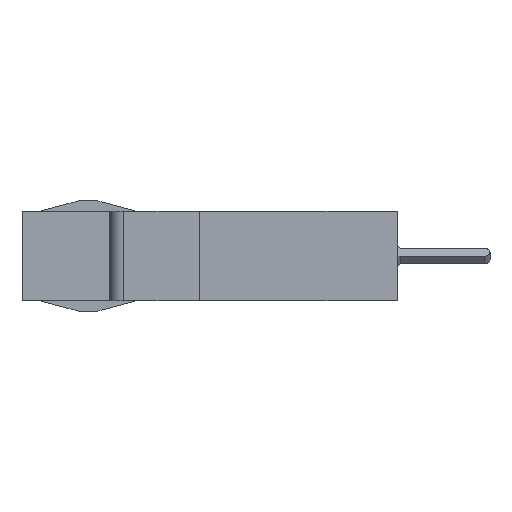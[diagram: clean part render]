
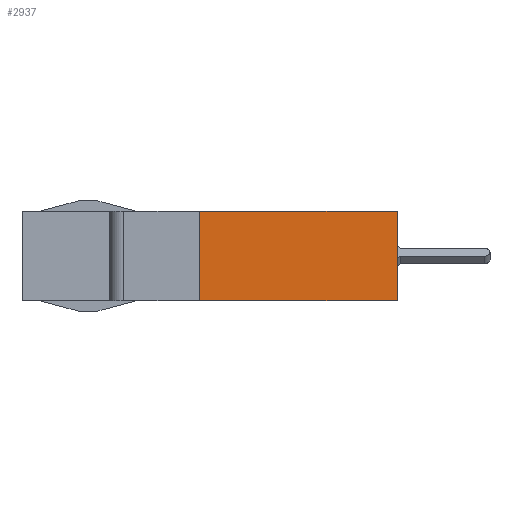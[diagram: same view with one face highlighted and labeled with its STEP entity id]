
A CAD part, left-side view. The second image highlights one B-rep face of the part: STEP entity #2937.
In plain terms, the highlighted planar face has unit normal (-1, 0, 0).
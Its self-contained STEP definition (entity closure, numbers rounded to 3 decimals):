
#182 = EDGE_CURVE ( 'NONE', #2905, #5426, #1135, .T. ) ;
#567 = DIRECTION ( 'NONE',  ( -1., 0., 0. ) ) ;
#622 = DIRECTION ( 'NONE',  ( 0., 0., 1. ) ) ;
#1115 = CARTESIAN_POINT ( 'NONE',  ( -2.235, 0., 2.54 ) ) ;
#1135 = LINE ( 'NONE', #4374, #2200 ) ;
#1329 = EDGE_CURVE ( 'NONE', #2905, #5324, #1978, .T. ) ;
#1419 = VECTOR ( 'NONE', #4460, 1000. ) ;
#1594 = DIRECTION ( 'NONE',  ( 0., 0., -1. ) ) ;
#1919 = CARTESIAN_POINT ( 'NONE',  ( -2.235, 0., -2.54 ) ) ;
#1951 = VERTEX_POINT ( 'NONE', #1115 ) ;
#1978 = LINE ( 'NONE', #3656, #1419 ) ;
#2200 = VECTOR ( 'NONE', #4913, 1000. ) ;
#2256 = EDGE_LOOP ( 'NONE', ( #5766, #2798, #2448, #4740 ) ) ;
#2448 = ORIENTED_EDGE ( 'NONE', *, *, #182, .F. ) ;
#2516 = EDGE_CURVE ( 'NONE', #5324, #1951, #4226, .T. ) ;
#2798 = ORIENTED_EDGE ( 'NONE', *, *, #5888, .T. ) ;
#2905 = VERTEX_POINT ( 'NONE', #5576 ) ;
#2937 = ADVANCED_FACE ( 'NONE', ( #6605 ), #5792, .T. ) ;
#3656 = CARTESIAN_POINT ( 'NONE',  ( -2.235, -11.176, -2.54 ) ) ;
#3705 = CARTESIAN_POINT ( 'NONE',  ( -2.235, -11.176, -2.54 ) ) ;
#4226 = LINE ( 'NONE', #4696, #4641 ) ;
#4374 = CARTESIAN_POINT ( 'NONE',  ( -2.235, -11.176, -2.54 ) ) ;
#4460 = DIRECTION ( 'NONE',  ( 0., 0., 1. ) ) ;
#4566 = AXIS2_PLACEMENT_3D ( 'NONE', #3705, #567, #622 ) ;
#4641 = VECTOR ( 'NONE', #5774, 1000. ) ;
#4696 = CARTESIAN_POINT ( 'NONE',  ( -2.235, -11.176, 2.54 ) ) ;
#4740 = ORIENTED_EDGE ( 'NONE', *, *, #1329, .T. ) ;
#4913 = DIRECTION ( 'NONE',  ( 0., 1., 0. ) ) ;
#5297 = CARTESIAN_POINT ( 'NONE',  ( -2.235, -11.176, 2.54 ) ) ;
#5324 = VERTEX_POINT ( 'NONE', #5297 ) ;
#5426 = VERTEX_POINT ( 'NONE', #1919 ) ;
#5576 = CARTESIAN_POINT ( 'NONE',  ( -2.235, -11.176, -2.54 ) ) ;
#5605 = CARTESIAN_POINT ( 'NONE',  ( -2.235, 0., 2.54 ) ) ;
#5766 = ORIENTED_EDGE ( 'NONE', *, *, #2516, .T. ) ;
#5774 = DIRECTION ( 'NONE',  ( 0., 1., 0. ) ) ;
#5792 = PLANE ( 'NONE',  #4566 ) ;
#5888 = EDGE_CURVE ( 'NONE', #1951, #5426, #6707, .T. ) ;
#6605 = FACE_OUTER_BOUND ( 'NONE', #2256, .T. ) ;
#6628 = VECTOR ( 'NONE', #1594, 1000. ) ;
#6707 = LINE ( 'NONE', #5605, #6628 ) ;
